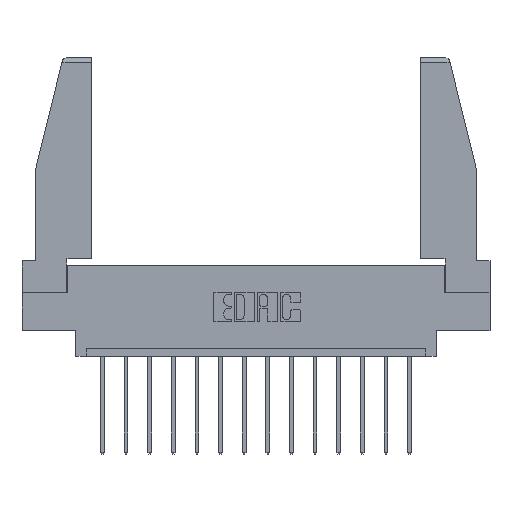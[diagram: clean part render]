
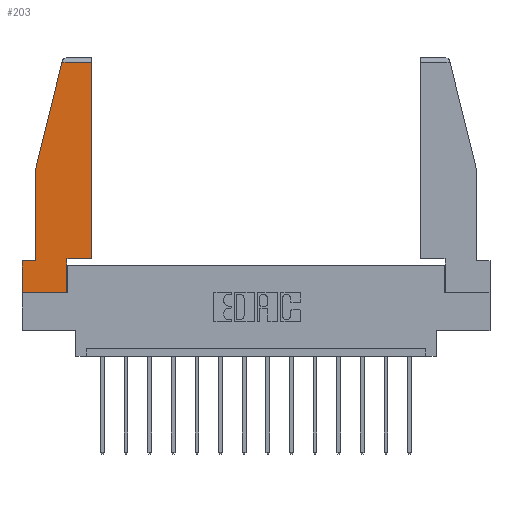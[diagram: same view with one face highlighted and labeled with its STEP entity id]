
A CAD part, top view. The second image highlights one B-rep face of the part: STEP entity #203.
In plain terms, the highlighted planar face has unit normal (0, 0, 1).
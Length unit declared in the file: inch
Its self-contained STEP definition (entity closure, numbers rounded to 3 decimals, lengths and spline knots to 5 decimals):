
#203 = ADVANCED_FACE ( 'NONE', ( #2075 ), #14197, .T. ) ;
#207 = VERTEX_POINT ( 'NONE', #10147 ) ;
#356 = VECTOR ( 'NONE', #12801, 39.37008 ) ;
#501 = ORIENTED_EDGE ( 'NONE', *, *, #3117, .T. ) ;
#869 = LINE ( 'NONE', #8021, #4238 ) ;
#1217 = ORIENTED_EDGE ( 'NONE', *, *, #1336, .T. ) ;
#1336 = EDGE_CURVE ( 'NONE', #9024, #207, #8577, .T. ) ;
#1479 = DIRECTION ( 'NONE',  ( -1., 0., 0. ) ) ;
#1798 = LINE ( 'NONE', #14085, #356 ) ;
#2075 = FACE_OUTER_BOUND ( 'NONE', #15881, .T. ) ;
#2124 = VECTOR ( 'NONE', #13058, 39.37008 ) ;
#2176 = VERTEX_POINT ( 'NONE', #13567 ) ;
#3117 = EDGE_CURVE ( 'NONE', #13908, #14223, #10140, .T. ) ;
#3144 = CARTESIAN_POINT ( 'NONE',  ( 0., 0.21, 0. ) ) ;
#3465 = LINE ( 'NONE', #11262, #10302 ) ;
#3676 = VECTOR ( 'NONE', #14712, 39.37008 ) ;
#3935 = VERTEX_POINT ( 'NONE', #6176 ) ;
#4031 = CARTESIAN_POINT ( 'NONE',  ( 0., 0., 0. ) ) ;
#4095 = CARTESIAN_POINT ( 'NONE',  ( 0.086, 0.21, 0. ) ) ;
#4238 = VECTOR ( 'NONE', #1479, 39.37008 ) ;
#5075 = CARTESIAN_POINT ( 'NONE',  ( 0.086, 0.8, 0. ) ) ;
#5457 = LINE ( 'NONE', #9004, #13917 ) ;
#5958 = CARTESIAN_POINT ( 'NONE',  ( 0.297, 0., 0. ) ) ;
#6092 = VECTOR ( 'NONE', #12756, 39.37008 ) ;
#6176 = CARTESIAN_POINT ( 'NONE',  ( 0.086, 0.8, 0. ) ) ;
#6395 = CARTESIAN_POINT ( 'NONE',  ( 0., 0., 0. ) ) ;
#6475 = CARTESIAN_POINT ( 'NONE',  ( 0., 1.52, 0. ) ) ;
#6635 = EDGE_CURVE ( 'NONE', #3935, #8827, #14193, .T. ) ;
#7367 = VECTOR ( 'NONE', #16557, 39.37008 ) ;
#8021 = CARTESIAN_POINT ( 'NONE',  ( 0., 0.21, 0. ) ) ;
#8577 = LINE ( 'NONE', #6475, #2124 ) ;
#8827 = VERTEX_POINT ( 'NONE', #4095 ) ;
#8929 = VERTEX_POINT ( 'NONE', #3144 ) ;
#9004 = CARTESIAN_POINT ( 'NONE',  ( 0.297, 0., 0. ) ) ;
#9024 = VERTEX_POINT ( 'NONE', #11096 ) ;
#9038 = EDGE_CURVE ( 'NONE', #9589, #2176, #12355, .T. ) ;
#9045 = ORIENTED_EDGE ( 'NONE', *, *, #6635, .T. ) ;
#9589 = VERTEX_POINT ( 'NONE', #14676 ) ;
#9775 = CARTESIAN_POINT ( 'NONE',  ( 0.297, 0.223, 0. ) ) ;
#9946 = EDGE_CURVE ( 'NONE', #8929, #13908, #10718, .T. ) ;
#10140 = LINE ( 'NONE', #11648, #6092 ) ;
#10147 = CARTESIAN_POINT ( 'NONE',  ( 0.2636, 1.52, 0. ) ) ;
#10302 = VECTOR ( 'NONE', #15400, 39.37008 ) ;
#10659 = EDGE_CURVE ( 'NONE', #8827, #8929, #869, .T. ) ;
#10718 = LINE ( 'NONE', #14651, #3676 ) ;
#10991 = DIRECTION ( 'NONE',  ( 1., 0., 0. ) ) ;
#11096 = CARTESIAN_POINT ( 'NONE',  ( 0.461, 1.52, 0. ) ) ;
#11262 = CARTESIAN_POINT ( 'NONE',  ( 0.461, 0.223, 0. ) ) ;
#11593 = DIRECTION ( 'NONE',  ( 1., 0., 0. ) ) ;
#11648 = CARTESIAN_POINT ( 'NONE',  ( 0., 0., 0. ) ) ;
#12355 = LINE ( 'NONE', #9775, #15569 ) ;
#12398 = EDGE_CURVE ( 'NONE', #207, #3935, #1798, .T. ) ;
#12756 = DIRECTION ( 'NONE',  ( 1., 0., 0. ) ) ;
#12801 = DIRECTION ( 'NONE',  ( -0.239, -0.971, 0. ) ) ;
#12803 = DIRECTION ( 'NONE',  ( 0., 0., 1. ) ) ;
#13058 = DIRECTION ( 'NONE',  ( -1., 0., 0. ) ) ;
#13567 = CARTESIAN_POINT ( 'NONE',  ( 0.461, 0.223, 0. ) ) ;
#13843 = ORIENTED_EDGE ( 'NONE', *, *, #9038, .T. ) ;
#13908 = VERTEX_POINT ( 'NONE', #6395 ) ;
#13917 = VECTOR ( 'NONE', #14053, 39.37008 ) ;
#14053 = DIRECTION ( 'NONE',  ( 0., 1., 0. ) ) ;
#14085 = CARTESIAN_POINT ( 'NONE',  ( 0.271, 1.55, 0. ) ) ;
#14193 = LINE ( 'NONE', #5075, #7367 ) ;
#14197 = PLANE ( 'NONE',  #16540 ) ;
#14223 = VERTEX_POINT ( 'NONE', #5958 ) ;
#14651 = CARTESIAN_POINT ( 'NONE',  ( 0., 0.21, 0. ) ) ;
#14676 = CARTESIAN_POINT ( 'NONE',  ( 0.297, 0.223, 0. ) ) ;
#14712 = DIRECTION ( 'NONE',  ( 0., -1., 0. ) ) ;
#14782 = ORIENTED_EDGE ( 'NONE', *, *, #15437, .T. ) ;
#14785 = ORIENTED_EDGE ( 'NONE', *, *, #12398, .T. ) ;
#14978 = ORIENTED_EDGE ( 'NONE', *, *, #9946, .T. ) ;
#15292 = ORIENTED_EDGE ( 'NONE', *, *, #16086, .T. ) ;
#15400 = DIRECTION ( 'NONE',  ( 0., 1., 0. ) ) ;
#15437 = EDGE_CURVE ( 'NONE', #14223, #9589, #5457, .T. ) ;
#15569 = VECTOR ( 'NONE', #10991, 39.37008 ) ;
#15881 = EDGE_LOOP ( 'NONE', ( #15292, #1217, #14785, #9045, #16643, #14978, #501, #14782, #13843 ) ) ;
#16086 = EDGE_CURVE ( 'NONE', #2176, #9024, #3465, .T. ) ;
#16540 = AXIS2_PLACEMENT_3D ( 'NONE', #4031, #12803, #11593 ) ;
#16557 = DIRECTION ( 'NONE',  ( 0., -1., 0. ) ) ;
#16643 = ORIENTED_EDGE ( 'NONE', *, *, #10659, .T. ) ;
